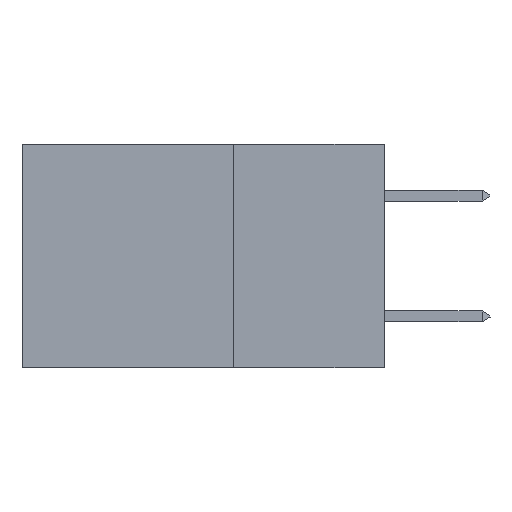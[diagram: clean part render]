
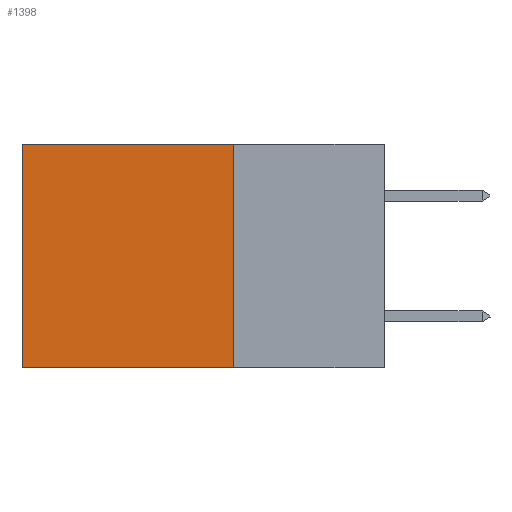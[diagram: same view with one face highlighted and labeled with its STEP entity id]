
A CAD part, left-side view. The second image highlights one B-rep face of the part: STEP entity #1398.
In plain terms, the highlighted planar face has unit normal (-1, 0, 0).
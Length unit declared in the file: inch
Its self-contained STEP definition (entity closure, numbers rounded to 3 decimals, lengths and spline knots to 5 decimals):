
#1398 = ADVANCED_FACE ( 'NONE', ( #5844 ), #21853, .F. ) ;
#1795 = VERTEX_POINT ( 'NONE', #5003 ) ;
#3398 = DIRECTION ( 'NONE',  ( 0., 0., -1. ) ) ;
#4546 = ORIENTED_EDGE ( 'NONE', *, *, #14426, .F. ) ;
#5003 = CARTESIAN_POINT ( 'NONE',  ( 0.2875, 0.6, -0.37 ) ) ;
#5844 = FACE_OUTER_BOUND ( 'NONE', #10322, .T. ) ;
#6166 = CARTESIAN_POINT ( 'NONE',  ( 0.2875, 0.25, -0.37 ) ) ;
#6826 = DIRECTION ( 'NONE',  ( 0., 1., 0. ) ) ;
#7514 = LINE ( 'NONE', #17625, #21279 ) ;
#7590 = CARTESIAN_POINT ( 'NONE',  ( 0.2875, 0.25, 0. ) ) ;
#10322 = EDGE_LOOP ( 'NONE', ( #16820, #4546, #25397, #23720 ) ) ;
#11371 = VECTOR ( 'NONE', #6826, 39.37008 ) ;
#11835 = DIRECTION ( 'NONE',  ( 0., 0., -1. ) ) ;
#12790 = AXIS2_PLACEMENT_3D ( 'NONE', #26022, #13803, #11835 ) ;
#13725 = EDGE_CURVE ( 'NONE', #19272, #22923, #16804, .T. ) ;
#13803 = DIRECTION ( 'NONE',  ( 1., 0., 0. ) ) ;
#13968 = EDGE_CURVE ( 'NONE', #22923, #1795, #7514, .T. ) ;
#14202 = VERTEX_POINT ( 'NONE', #6166 ) ;
#14426 = EDGE_CURVE ( 'NONE', #14202, #1795, #15182, .T. ) ;
#14451 = LINE ( 'NONE', #7590, #22469 ) ;
#14685 = CARTESIAN_POINT ( 'NONE',  ( 0.2875, 0.25, 0. ) ) ;
#15182 = LINE ( 'NONE', #22715, #20598 ) ;
#16804 = LINE ( 'NONE', #19059, #11371 ) ;
#16820 = ORIENTED_EDGE ( 'NONE', *, *, #13968, .T. ) ;
#17625 = CARTESIAN_POINT ( 'NONE',  ( 0.2875, 0.6, 0. ) ) ;
#19059 = CARTESIAN_POINT ( 'NONE',  ( 0.2875, 0.25, 0. ) ) ;
#19272 = VERTEX_POINT ( 'NONE', #14685 ) ;
#20598 = VECTOR ( 'NONE', #23441, 39.37008 ) ;
#20961 = CARTESIAN_POINT ( 'NONE',  ( 0.2875, 0.6, 0. ) ) ;
#21279 = VECTOR ( 'NONE', #3398, 39.37008 ) ;
#21853 = PLANE ( 'NONE',  #12790 ) ;
#21904 = DIRECTION ( 'NONE',  ( 0., 0., -1. ) ) ;
#22469 = VECTOR ( 'NONE', #21904, 39.37008 ) ;
#22715 = CARTESIAN_POINT ( 'NONE',  ( 0.2875, 0.25, -0.37 ) ) ;
#22923 = VERTEX_POINT ( 'NONE', #20961 ) ;
#23441 = DIRECTION ( 'NONE',  ( 0., 1., 0. ) ) ;
#23720 = ORIENTED_EDGE ( 'NONE', *, *, #13725, .T. ) ;
#23825 = EDGE_CURVE ( 'NONE', #19272, #14202, #14451, .T. ) ;
#25397 = ORIENTED_EDGE ( 'NONE', *, *, #23825, .F. ) ;
#26022 = CARTESIAN_POINT ( 'NONE',  ( 0.2875, 0.25, 0. ) ) ;
